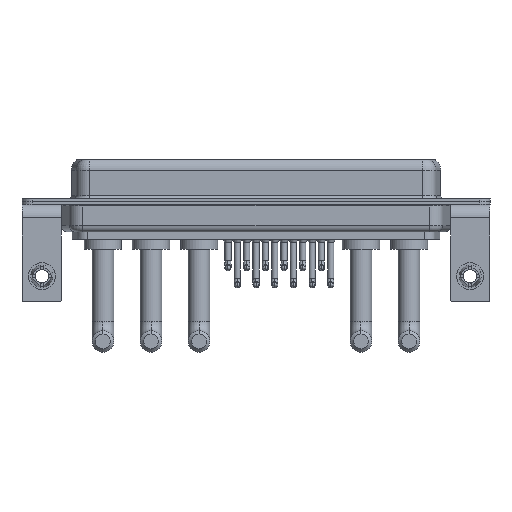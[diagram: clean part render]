
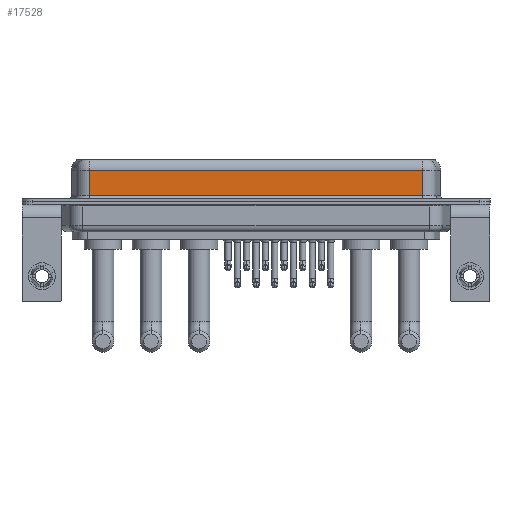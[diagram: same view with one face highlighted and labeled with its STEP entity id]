
A CAD part, front view. The second image highlights one B-rep face of the part: STEP entity #17528.
In plain terms, the highlighted planar face has unit normal (0, -1, 0).
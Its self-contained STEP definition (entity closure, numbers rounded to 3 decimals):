
#183 = VERTEX_POINT ( 'NONE', #652 ) ;
#415 = PLANE ( 'NONE',  #5827 ) ;
#652 = CARTESIAN_POINT ( 'NONE',  ( 7.038, -3.95, 4.65 ) ) ;
#1316 = LINE ( 'NONE', #17005, #13607 ) ;
#1775 = EDGE_CURVE ( 'NONE', #11148, #183, #22170, .T. ) ;
#5052 = CARTESIAN_POINT ( 'NONE',  ( 7.038, -3.95, 6.4 ) ) ;
#5407 = CARTESIAN_POINT ( 'NONE',  ( 56.462, -3.95, 0.9 ) ) ;
#5757 = ORIENTED_EDGE ( 'NONE', *, *, #19533, .F. ) ;
#5827 = AXIS2_PLACEMENT_3D ( 'NONE', #12572, #18051, #21465 ) ;
#6492 = DIRECTION ( 'NONE',  ( -1., 0., 0. ) ) ;
#8099 = CARTESIAN_POINT ( 'NONE',  ( 56.462, -3.95, 4.65 ) ) ;
#9179 = DIRECTION ( 'NONE',  ( 1., 0., 0. ) ) ;
#9752 = CARTESIAN_POINT ( 'NONE',  ( 56.462, -3.95, 0.9 ) ) ;
#10656 = ORIENTED_EDGE ( 'NONE', *, *, #11892, .T. ) ;
#11057 = ORIENTED_EDGE ( 'NONE', *, *, #1775, .T. ) ;
#11148 = VERTEX_POINT ( 'NONE', #18752 ) ;
#11189 = FACE_OUTER_BOUND ( 'NONE', #11191, .T. ) ;
#11191 = EDGE_LOOP ( 'NONE', ( #5757, #11057, #14728, #10656 ) ) ;
#11339 = CARTESIAN_POINT ( 'NONE',  ( 7.038, -3.95, 0.9 ) ) ;
#11892 = EDGE_CURVE ( 'NONE', #17063, #16805, #17884, .T. ) ;
#12054 = DIRECTION ( 'NONE',  ( 0., 0., -1. ) ) ;
#12572 = CARTESIAN_POINT ( 'NONE',  ( 56.462, -3.95, 6.4 ) ) ;
#13607 = VECTOR ( 'NONE', #15279, 1000. ) ;
#13769 = LINE ( 'NONE', #5052, #19101 ) ;
#14728 = ORIENTED_EDGE ( 'NONE', *, *, #20181, .T. ) ;
#15265 = VECTOR ( 'NONE', #9179, 1000. ) ;
#15279 = DIRECTION ( 'NONE',  ( 0., 0., -1. ) ) ;
#16805 = VERTEX_POINT ( 'NONE', #9752 ) ;
#17005 = CARTESIAN_POINT ( 'NONE',  ( 56.462, -3.95, 6.4 ) ) ;
#17063 = VERTEX_POINT ( 'NONE', #11339 ) ;
#17528 = ADVANCED_FACE ( 'NONE', ( #11189 ), #415, .F. ) ;
#17884 = LINE ( 'NONE', #5407, #15265 ) ;
#18051 = DIRECTION ( 'NONE',  ( 0., 1., 0. ) ) ;
#18752 = CARTESIAN_POINT ( 'NONE',  ( 56.462, -3.95, 4.65 ) ) ;
#19101 = VECTOR ( 'NONE', #12054, 1000. ) ;
#19533 = EDGE_CURVE ( 'NONE', #11148, #16805, #1316, .T. ) ;
#20181 = EDGE_CURVE ( 'NONE', #183, #17063, #13769, .T. ) ;
#21465 = DIRECTION ( 'NONE',  ( 0., 0., 1. ) ) ;
#21965 = VECTOR ( 'NONE', #6492, 1000. ) ;
#22170 = LINE ( 'NONE', #8099, #21965 ) ;
